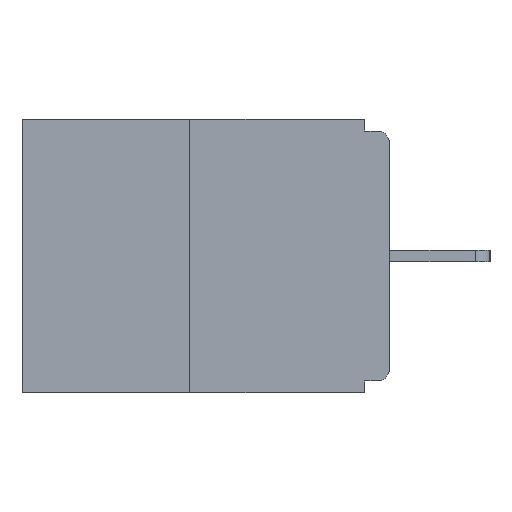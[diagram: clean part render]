
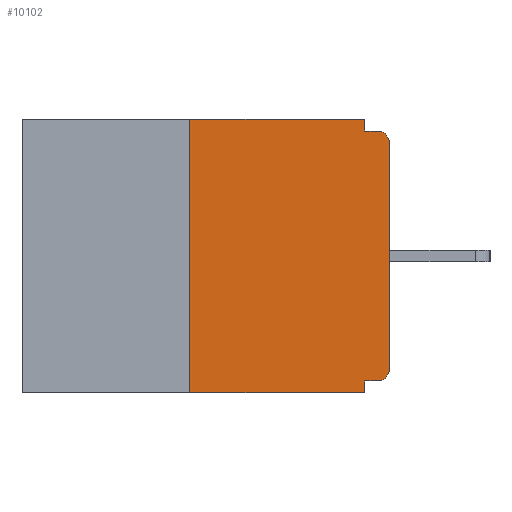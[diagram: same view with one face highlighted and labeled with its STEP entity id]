
A CAD part, left-side view. The second image highlights one B-rep face of the part: STEP entity #10102.
In plain terms, the highlighted planar face has unit normal (-1, 0, 0).
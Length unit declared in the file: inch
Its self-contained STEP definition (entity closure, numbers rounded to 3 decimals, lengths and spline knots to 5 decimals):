
#245 = LINE ( 'NONE', #19678, #4422 ) ;
#619 = CARTESIAN_POINT ( 'NONE',  ( 0., 0., -0.03 ) ) ;
#955 = EDGE_CURVE ( 'NONE', #19808, #18758, #1303, .T. ) ;
#1079 = ORIENTED_EDGE ( 'NONE', *, *, #11429, .T. ) ;
#1303 = LINE ( 'NONE', #4958, #22113 ) ;
#1398 = EDGE_CURVE ( 'NONE', #5210, #15006, #12818, .T. ) ;
#1461 = CIRCLE ( 'NONE', #11205, 0.015 ) ;
#1842 = CARTESIAN_POINT ( 'NONE',  ( 0., 0.031, -0.328 ) ) ;
#1856 = DIRECTION ( 'NONE',  ( 0., 0., -1. ) ) ;
#2038 = VECTOR ( 'NONE', #13665, 39.37008 ) ;
#2077 = ORIENTED_EDGE ( 'NONE', *, *, #4505, .F. ) ;
#2938 = DIRECTION ( 'NONE',  ( 0., -1., 0. ) ) ;
#4401 = LINE ( 'NONE', #19661, #6840 ) ;
#4422 = VECTOR ( 'NONE', #19558, 39.37008 ) ;
#4505 = EDGE_CURVE ( 'NONE', #24985, #25074, #16335, .T. ) ;
#4595 = CARTESIAN_POINT ( 'NONE',  ( 0., 0.25, -0.343 ) ) ;
#4944 = CARTESIAN_POINT ( 'NONE',  ( 0., 0.015, -0.03 ) ) ;
#4958 = CARTESIAN_POINT ( 'NONE',  ( 0., 0., 0. ) ) ;
#5210 = VERTEX_POINT ( 'NONE', #1842 ) ;
#5214 = AXIS2_PLACEMENT_3D ( 'NONE', #17336, #17693, #1856 ) ;
#5439 = FACE_OUTER_BOUND ( 'NONE', #8694, .T. ) ;
#5687 = DIRECTION ( 'NONE',  ( 0., 0., -1. ) ) ;
#6038 = ORIENTED_EDGE ( 'NONE', *, *, #1398, .F. ) ;
#6800 = ORIENTED_EDGE ( 'NONE', *, *, #7208, .F. ) ;
#6840 = VECTOR ( 'NONE', #19921, 39.37008 ) ;
#6961 = CARTESIAN_POINT ( 'NONE',  ( 0., 0.031, -0.343 ) ) ;
#7104 = DIRECTION ( 'NONE',  ( -1., 0., 0. ) ) ;
#7208 = EDGE_CURVE ( 'NONE', #25074, #11760, #16375, .T. ) ;
#7350 = CARTESIAN_POINT ( 'NONE',  ( 0., 0.46, 0. ) ) ;
#7468 = PLANE ( 'NONE',  #22940 ) ;
#7897 = CARTESIAN_POINT ( 'NONE',  ( 0., 0.031, -0.343 ) ) ;
#8191 = EDGE_CURVE ( 'NONE', #19239, #14654, #20590, .T. ) ;
#8301 = CARTESIAN_POINT ( 'NONE',  ( 0., 0.031, 0. ) ) ;
#8694 = EDGE_LOOP ( 'NONE', ( #6800, #2077, #1079, #6038, #13914, #9087, #18915, #9219, #24999, #23767 ) ) ;
#8741 = DIRECTION ( 'NONE',  ( 0., 0., -1. ) ) ;
#8826 = CARTESIAN_POINT ( 'NONE',  ( 0., 0.015, -0.328 ) ) ;
#9087 = ORIENTED_EDGE ( 'NONE', *, *, #23599, .T. ) ;
#9219 = ORIENTED_EDGE ( 'NONE', *, *, #15939, .T. ) ;
#10102 = ADVANCED_FACE ( 'NONE', ( #5439 ), #7468, .F. ) ;
#10368 = CARTESIAN_POINT ( 'NONE',  ( 0., 0.031, -0.015 ) ) ;
#10380 = DIRECTION ( 'NONE',  ( 0., 0., 1. ) ) ;
#11205 = AXIS2_PLACEMENT_3D ( 'NONE', #4944, #7104, #14862 ) ;
#11429 = EDGE_CURVE ( 'NONE', #24985, #15006, #4401, .T. ) ;
#11760 = VERTEX_POINT ( 'NONE', #8301 ) ;
#12010 = CARTESIAN_POINT ( 'NONE',  ( 0., 0.015, -0.015 ) ) ;
#12818 = LINE ( 'NONE', #6961, #13210 ) ;
#13210 = VECTOR ( 'NONE', #8741, 39.37008 ) ;
#13665 = DIRECTION ( 'NONE',  ( 0., 0., -1. ) ) ;
#13914 = ORIENTED_EDGE ( 'NONE', *, *, #18571, .F. ) ;
#14253 = VECTOR ( 'NONE', #22361, 39.37008 ) ;
#14612 = CARTESIAN_POINT ( 'NONE',  ( 0., 0., -0.015 ) ) ;
#14654 = VERTEX_POINT ( 'NONE', #12010 ) ;
#14862 = DIRECTION ( 'NONE',  ( 0., 0., -1. ) ) ;
#15006 = VERTEX_POINT ( 'NONE', #7897 ) ;
#15466 = LINE ( 'NONE', #19170, #2038 ) ;
#15939 = EDGE_CURVE ( 'NONE', #18758, #14654, #1461, .T. ) ;
#16335 = LINE ( 'NONE', #20033, #20232 ) ;
#16375 = LINE ( 'NONE', #20710, #18373 ) ;
#17336 = CARTESIAN_POINT ( 'NONE',  ( 0., 0.015, -0.313 ) ) ;
#17693 = DIRECTION ( 'NONE',  ( -1., 0., 0. ) ) ;
#18373 = VECTOR ( 'NONE', #2938, 39.37008 ) ;
#18571 = EDGE_CURVE ( 'NONE', #24471, #5210, #245, .T. ) ;
#18758 = VERTEX_POINT ( 'NONE', #619 ) ;
#18915 = ORIENTED_EDGE ( 'NONE', *, *, #955, .T. ) ;
#18976 = CARTESIAN_POINT ( 'NONE',  ( 0., 0., -0.313 ) ) ;
#19039 = EDGE_CURVE ( 'NONE', #11760, #19239, #15466, .T. ) ;
#19170 = CARTESIAN_POINT ( 'NONE',  ( 0., 0.031, 0. ) ) ;
#19239 = VERTEX_POINT ( 'NONE', #10368 ) ;
#19558 = DIRECTION ( 'NONE',  ( 0., 1., 0. ) ) ;
#19661 = CARTESIAN_POINT ( 'NONE',  ( 0., 0.46, -0.343 ) ) ;
#19678 = CARTESIAN_POINT ( 'NONE',  ( 0., 0., -0.328 ) ) ;
#19808 = VERTEX_POINT ( 'NONE', #18976 ) ;
#19921 = DIRECTION ( 'NONE',  ( 0., -1., 0. ) ) ;
#20033 = CARTESIAN_POINT ( 'NONE',  ( 0., 0.25, 0. ) ) ;
#20211 = CIRCLE ( 'NONE', #5214, 0.015 ) ;
#20232 = VECTOR ( 'NONE', #10380, 39.37008 ) ;
#20473 = DIRECTION ( 'NONE',  ( 0., 0., 1. ) ) ;
#20590 = LINE ( 'NONE', #14612, #14253 ) ;
#20710 = CARTESIAN_POINT ( 'NONE',  ( 0., 0.46, 0. ) ) ;
#22113 = VECTOR ( 'NONE', #20473, 39.37008 ) ;
#22361 = DIRECTION ( 'NONE',  ( 0., -1., 0. ) ) ;
#22940 = AXIS2_PLACEMENT_3D ( 'NONE', #7350, #23092, #5687 ) ;
#23092 = DIRECTION ( 'NONE',  ( 1., 0., 0. ) ) ;
#23599 = EDGE_CURVE ( 'NONE', #24471, #19808, #20211, .T. ) ;
#23767 = ORIENTED_EDGE ( 'NONE', *, *, #19039, .F. ) ;
#24471 = VERTEX_POINT ( 'NONE', #8826 ) ;
#24539 = CARTESIAN_POINT ( 'NONE',  ( 0., 0.25, 0. ) ) ;
#24985 = VERTEX_POINT ( 'NONE', #4595 ) ;
#24999 = ORIENTED_EDGE ( 'NONE', *, *, #8191, .F. ) ;
#25074 = VERTEX_POINT ( 'NONE', #24539 ) ;
